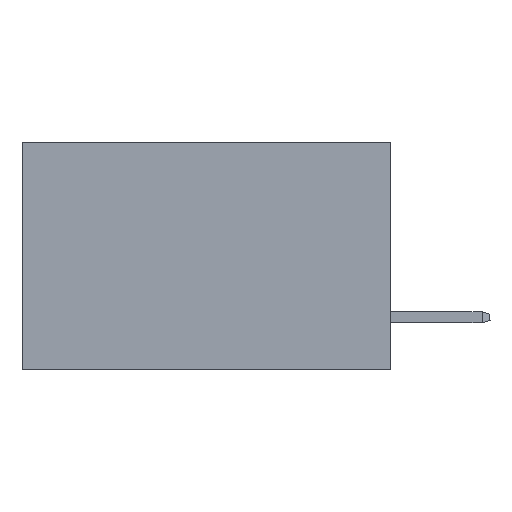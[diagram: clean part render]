
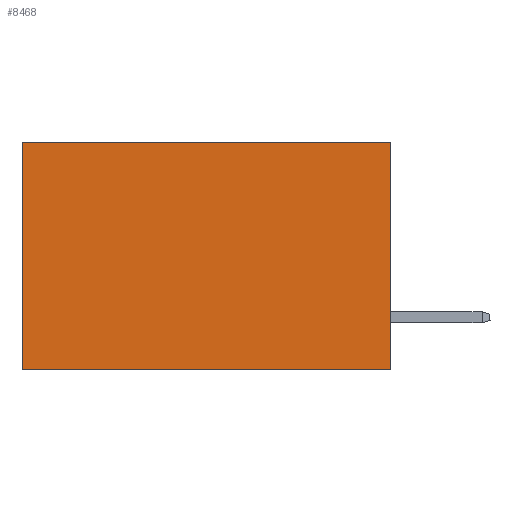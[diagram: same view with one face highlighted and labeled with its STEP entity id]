
A CAD part, left-side view. The second image highlights one B-rep face of the part: STEP entity #8468.
In plain terms, the highlighted planar face has unit normal (-1, 0, 0).
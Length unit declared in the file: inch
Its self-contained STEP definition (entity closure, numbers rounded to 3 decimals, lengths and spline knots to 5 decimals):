
#716 = EDGE_CURVE ( 'NONE', #2622, #6358, #15401, .T. ) ;
#1386 = CARTESIAN_POINT ( 'NONE',  ( 0.2875, 0.6, 0. ) ) ;
#1560 = CARTESIAN_POINT ( 'NONE',  ( 0.2875, 0., -0.37 ) ) ;
#1801 = VECTOR ( 'NONE', #5505, 39.37008 ) ;
#2622 = VERTEX_POINT ( 'NONE', #12197 ) ;
#3640 = LINE ( 'NONE', #3877, #15210 ) ;
#3877 = CARTESIAN_POINT ( 'NONE',  ( 0.2875, 0., 0. ) ) ;
#5024 = LINE ( 'NONE', #1560, #7997 ) ;
#5252 = DIRECTION ( 'NONE',  ( 0., 1., 0. ) ) ;
#5393 = VERTEX_POINT ( 'NONE', #12360 ) ;
#5505 = DIRECTION ( 'NONE',  ( 0., 1., 0. ) ) ;
#5653 = CARTESIAN_POINT ( 'NONE',  ( 0.2875, 0.6, 0. ) ) ;
#6037 = CARTESIAN_POINT ( 'NONE',  ( 0.2875, 0., 0. ) ) ;
#6134 = ORIENTED_EDGE ( 'NONE', *, *, #716, .T. ) ;
#6286 = EDGE_CURVE ( 'NONE', #2622, #5393, #3640, .T. ) ;
#6358 = VERTEX_POINT ( 'NONE', #1386 ) ;
#7997 = VECTOR ( 'NONE', #5252, 39.37008 ) ;
#8435 = LINE ( 'NONE', #5653, #13836 ) ;
#8468 = ADVANCED_FACE ( 'NONE', ( #15342 ), #14948, .F. ) ;
#8593 = DIRECTION ( 'NONE',  ( 0., 0., -1. ) ) ;
#10031 = ORIENTED_EDGE ( 'NONE', *, *, #12495, .T. ) ;
#10758 = CARTESIAN_POINT ( 'NONE',  ( 0.2875, 0.6, -0.37 ) ) ;
#10982 = AXIS2_PLACEMENT_3D ( 'NONE', #6037, #11040, #8593 ) ;
#11040 = DIRECTION ( 'NONE',  ( 1., 0., 0. ) ) ;
#11171 = VERTEX_POINT ( 'NONE', #10758 ) ;
#12011 = EDGE_LOOP ( 'NONE', ( #10031, #12084, #13350, #6134 ) ) ;
#12084 = ORIENTED_EDGE ( 'NONE', *, *, #14234, .F. ) ;
#12197 = CARTESIAN_POINT ( 'NONE',  ( 0.2875, 0., 0. ) ) ;
#12360 = CARTESIAN_POINT ( 'NONE',  ( 0.2875, 0., -0.37 ) ) ;
#12495 = EDGE_CURVE ( 'NONE', #6358, #11171, #8435, .T. ) ;
#12787 = DIRECTION ( 'NONE',  ( 0., 0., -1. ) ) ;
#13350 = ORIENTED_EDGE ( 'NONE', *, *, #6286, .F. ) ;
#13465 = DIRECTION ( 'NONE',  ( 0., 0., -1. ) ) ;
#13836 = VECTOR ( 'NONE', #13465, 39.37008 ) ;
#14234 = EDGE_CURVE ( 'NONE', #5393, #11171, #5024, .T. ) ;
#14369 = CARTESIAN_POINT ( 'NONE',  ( 0.2875, 0., 0. ) ) ;
#14948 = PLANE ( 'NONE',  #10982 ) ;
#15210 = VECTOR ( 'NONE', #12787, 39.37008 ) ;
#15342 = FACE_OUTER_BOUND ( 'NONE', #12011, .T. ) ;
#15401 = LINE ( 'NONE', #14369, #1801 ) ;
